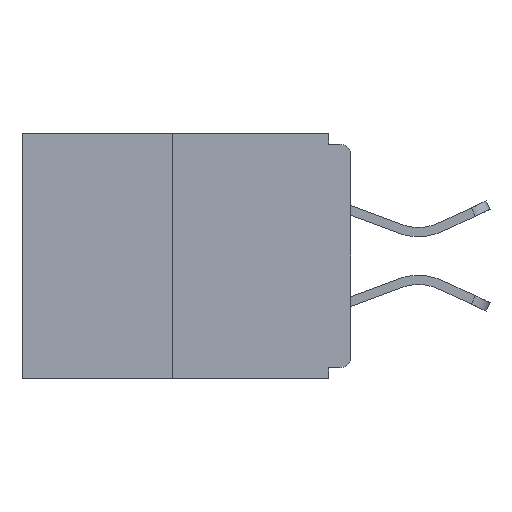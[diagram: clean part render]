
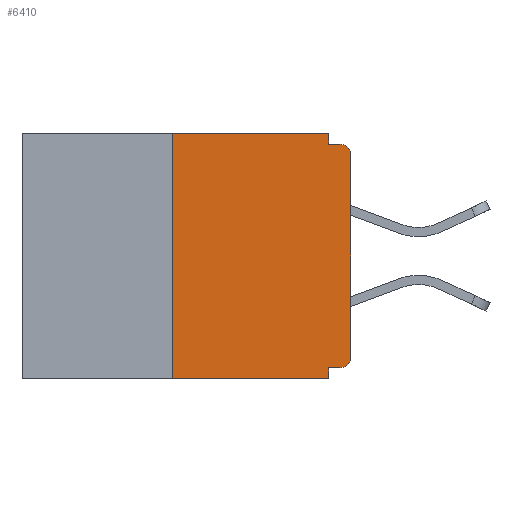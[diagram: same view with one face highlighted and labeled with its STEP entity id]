
A CAD part, left-side view. The second image highlights one B-rep face of the part: STEP entity #6410.
In plain terms, the highlighted planar face has unit normal (-1, 0, 0).
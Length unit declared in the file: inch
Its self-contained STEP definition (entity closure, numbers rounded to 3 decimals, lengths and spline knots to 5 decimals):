
#235 = LINE ( 'NONE', #15683, #19342 ) ;
#240 = EDGE_CURVE ( 'NONE', #12504, #17840, #15397, .T. ) ;
#584 = EDGE_CURVE ( 'NONE', #17840, #7731, #7203, .T. ) ;
#619 = EDGE_LOOP ( 'NONE', ( #12191, #14501, #14449, #17414, #4401, #9389, #6082, #14003, #13925, #13087 ) ) ;
#1084 = DIRECTION ( 'NONE',  ( 0., 1., 0. ) ) ;
#1144 = AXIS2_PLACEMENT_3D ( 'NONE', #14815, #9702, #16234 ) ;
#1273 = LINE ( 'NONE', #7609, #15840 ) ;
#1431 = AXIS2_PLACEMENT_3D ( 'NONE', #13426, #5747, #12314 ) ;
#1920 = CARTESIAN_POINT ( 'NONE',  ( 0., 0., -0.03 ) ) ;
#2147 = VERTEX_POINT ( 'NONE', #14341 ) ;
#2297 = LINE ( 'NONE', #12950, #13276 ) ;
#2636 = CARTESIAN_POINT ( 'NONE',  ( 0., 0., -0.328 ) ) ;
#2748 = DIRECTION ( 'NONE',  ( 0., 0., -1. ) ) ;
#3777 = DIRECTION ( 'NONE',  ( 1., 0., 0. ) ) ;
#4077 = CARTESIAN_POINT ( 'NONE',  ( 0., 0.46, 0. ) ) ;
#4401 = ORIENTED_EDGE ( 'NONE', *, *, #17925, .F. ) ;
#5493 = CARTESIAN_POINT ( 'NONE',  ( 0., 0.031, -0.343 ) ) ;
#5701 = FACE_OUTER_BOUND ( 'NONE', #619, .T. ) ;
#5747 = DIRECTION ( 'NONE',  ( -1., 0., 0. ) ) ;
#5888 = CARTESIAN_POINT ( 'NONE',  ( 0., 0., 0. ) ) ;
#6082 = ORIENTED_EDGE ( 'NONE', *, *, #12716, .T. ) ;
#6410 = ADVANCED_FACE ( 'NONE', ( #5701 ), #18060, .F. ) ;
#6756 = VECTOR ( 'NONE', #2748, 39.37008 ) ;
#7161 = EDGE_CURVE ( 'NONE', #18417, #8821, #235, .T. ) ;
#7203 = LINE ( 'NONE', #18225, #14550 ) ;
#7376 = VECTOR ( 'NONE', #7904, 39.37008 ) ;
#7403 = DIRECTION ( 'NONE',  ( 0., -1., 0. ) ) ;
#7422 = CARTESIAN_POINT ( 'NONE',  ( 0., 0.25, -0.343 ) ) ;
#7609 = CARTESIAN_POINT ( 'NONE',  ( 0., 0.25, 0. ) ) ;
#7731 = VERTEX_POINT ( 'NONE', #12919 ) ;
#7904 = DIRECTION ( 'NONE',  ( 0., 0., -1. ) ) ;
#7939 = EDGE_CURVE ( 'NONE', #16246, #7731, #16123, .T. ) ;
#8575 = CARTESIAN_POINT ( 'NONE',  ( 0., 0.25, 0. ) ) ;
#8741 = EDGE_CURVE ( 'NONE', #2147, #12291, #15510, .T. ) ;
#8821 = VERTEX_POINT ( 'NONE', #5493 ) ;
#9337 = EDGE_CURVE ( 'NONE', #18417, #11057, #1273, .T. ) ;
#9389 = ORIENTED_EDGE ( 'NONE', *, *, #8741, .T. ) ;
#9692 = AXIS2_PLACEMENT_3D ( 'NONE', #4077, #3777, #17965 ) ;
#9702 = DIRECTION ( 'NONE',  ( -1., 0., 0. ) ) ;
#10287 = VERTEX_POINT ( 'NONE', #19648 ) ;
#11057 = VERTEX_POINT ( 'NONE', #8575 ) ;
#11352 = VECTOR ( 'NONE', #12157, 39.37008 ) ;
#11542 = CARTESIAN_POINT ( 'NONE',  ( 0., 0.031, -0.015 ) ) ;
#11735 = DIRECTION ( 'NONE',  ( 0., -1., 0. ) ) ;
#12157 = DIRECTION ( 'NONE',  ( 0., 0., 1. ) ) ;
#12191 = ORIENTED_EDGE ( 'NONE', *, *, #18202, .F. ) ;
#12209 = EDGE_CURVE ( 'NONE', #10287, #8821, #19907, .T. ) ;
#12291 = VERTEX_POINT ( 'NONE', #13607 ) ;
#12314 = DIRECTION ( 'NONE',  ( 0., 0., -1. ) ) ;
#12504 = VERTEX_POINT ( 'NONE', #13286 ) ;
#12716 = EDGE_CURVE ( 'NONE', #12291, #16246, #19886, .T. ) ;
#12919 = CARTESIAN_POINT ( 'NONE',  ( 0., 0.015, -0.015 ) ) ;
#12950 = CARTESIAN_POINT ( 'NONE',  ( 0., 0.46, 0. ) ) ;
#13087 = ORIENTED_EDGE ( 'NONE', *, *, #240, .F. ) ;
#13276 = VECTOR ( 'NONE', #11735, 39.37008 ) ;
#13286 = CARTESIAN_POINT ( 'NONE',  ( 0., 0.031, 0. ) ) ;
#13426 = CARTESIAN_POINT ( 'NONE',  ( 0., 0.015, -0.03 ) ) ;
#13607 = CARTESIAN_POINT ( 'NONE',  ( 0., 0., -0.313 ) ) ;
#13862 = CARTESIAN_POINT ( 'NONE',  ( 0., 0.031, 0. ) ) ;
#13925 = ORIENTED_EDGE ( 'NONE', *, *, #584, .F. ) ;
#14003 = ORIENTED_EDGE ( 'NONE', *, *, #7939, .T. ) ;
#14161 = DIRECTION ( 'NONE',  ( 0., -1., 0. ) ) ;
#14341 = CARTESIAN_POINT ( 'NONE',  ( 0., 0.015, -0.328 ) ) ;
#14449 = ORIENTED_EDGE ( 'NONE', *, *, #7161, .T. ) ;
#14501 = ORIENTED_EDGE ( 'NONE', *, *, #9337, .F. ) ;
#14550 = VECTOR ( 'NONE', #7403, 39.37008 ) ;
#14815 = CARTESIAN_POINT ( 'NONE',  ( 0., 0.015, -0.313 ) ) ;
#14938 = VECTOR ( 'NONE', #1084, 39.37008 ) ;
#15397 = LINE ( 'NONE', #13862, #7376 ) ;
#15510 = CIRCLE ( 'NONE', #1144, 0.015 ) ;
#15683 = CARTESIAN_POINT ( 'NONE',  ( 0., 0.46, -0.343 ) ) ;
#15840 = VECTOR ( 'NONE', #19958, 39.37008 ) ;
#16123 = CIRCLE ( 'NONE', #1431, 0.015 ) ;
#16234 = DIRECTION ( 'NONE',  ( 0., 0., -1. ) ) ;
#16246 = VERTEX_POINT ( 'NONE', #1920 ) ;
#17414 = ORIENTED_EDGE ( 'NONE', *, *, #12209, .F. ) ;
#17840 = VERTEX_POINT ( 'NONE', #11542 ) ;
#17925 = EDGE_CURVE ( 'NONE', #2147, #10287, #18470, .T. ) ;
#17965 = DIRECTION ( 'NONE',  ( 0., 0., -1. ) ) ;
#18060 = PLANE ( 'NONE',  #9692 ) ;
#18202 = EDGE_CURVE ( 'NONE', #11057, #12504, #2297, .T. ) ;
#18225 = CARTESIAN_POINT ( 'NONE',  ( 0., 0., -0.015 ) ) ;
#18417 = VERTEX_POINT ( 'NONE', #7422 ) ;
#18470 = LINE ( 'NONE', #2636, #14938 ) ;
#18493 = CARTESIAN_POINT ( 'NONE',  ( 0., 0.031, -0.343 ) ) ;
#19342 = VECTOR ( 'NONE', #14161, 39.37008 ) ;
#19648 = CARTESIAN_POINT ( 'NONE',  ( 0., 0.031, -0.328 ) ) ;
#19886 = LINE ( 'NONE', #5888, #11352 ) ;
#19907 = LINE ( 'NONE', #18493, #6756 ) ;
#19958 = DIRECTION ( 'NONE',  ( 0., 0., 1. ) ) ;
